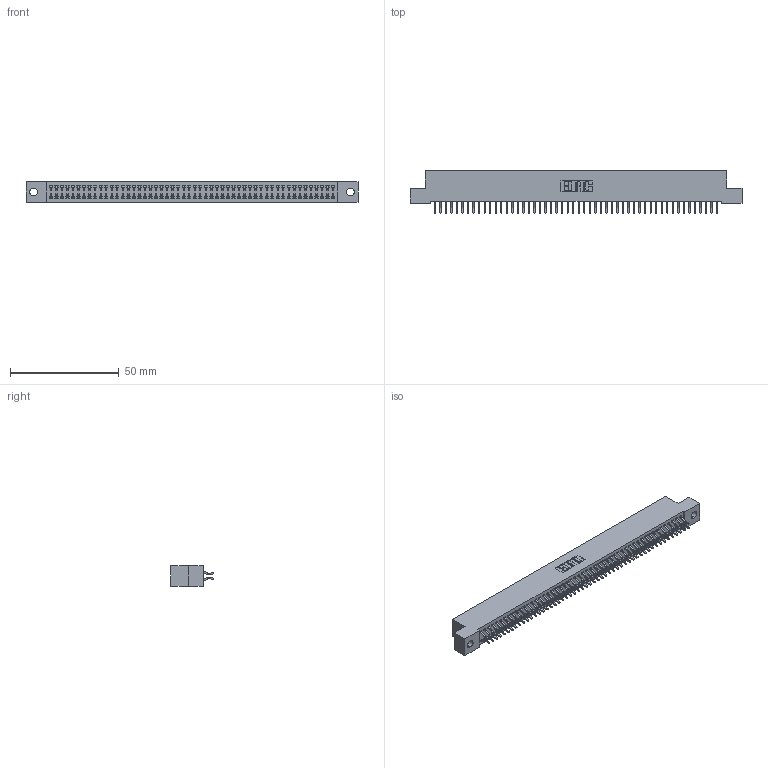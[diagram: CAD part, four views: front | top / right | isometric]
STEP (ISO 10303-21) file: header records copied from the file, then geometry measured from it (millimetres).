
FILE_DESCRIPTION (( 'STEP AP203' ), '1' );
FILE_NAME ('342-104-556-202.STEP', '2018-08-14T06:23:23', ( '' ), ( '' ), 'SwSTEP 2.0', 'SolidWorks 2016', '' );
FILE_SCHEMA (( 'CONFIG_CONTROL_DESIGN' ));
Length unit declared in the file: inch
Products named in the file (3): 345-292-001_556 Tail; 342-104-556-202; 342 Part_.128 Slot
Assembly tree (105 placements, depth 2):
  342-104-556-202
    342 Part_.128 Slot
    345-292-001_556 Tail  x104
Bounding box: 152.4 x 19.58 x 9.4 mm (x, y, z)
Volume: 13685.7 mm3; surface area: 22181.8 mm2
Topology: 105 solids, 105 shells, 6146 faces, 18303 edges, 12062 vertices
Faces by surface type: plane 4230, cylinder 1916
Entity records: 32383 total; most frequent: CARTESIAN_POINT 5370, ORIENTED_EDGE 5294, DIRECTION 4559, EDGE_CURVE 2647, VECTOR 2511, LINE 2511, VERTEX_POINT 1762, AXIS2_PLACEMENT_3D 1024
